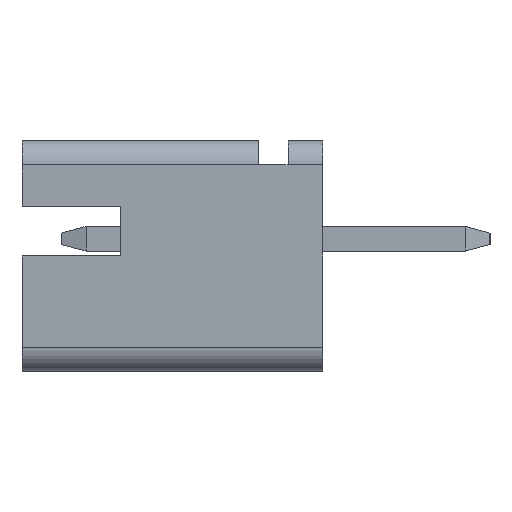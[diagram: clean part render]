
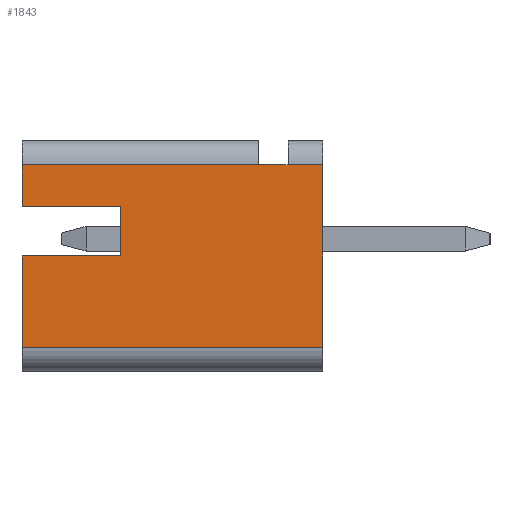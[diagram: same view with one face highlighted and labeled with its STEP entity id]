
A CAD part, left-side view. The second image highlights one B-rep face of the part: STEP entity #1843.
In plain terms, the highlighted planar face has unit normal (-1, 0, 0).
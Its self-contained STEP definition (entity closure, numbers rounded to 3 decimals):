
#8 = CARTESIAN_POINT ( 'NONE',  ( -2., 6.1, -0.35 ) ) ;
#12 = ORIENTED_EDGE ( 'NONE', *, *, #127, .F. ) ;
#119 = LINE ( 'NONE', #939, #4665 ) ;
#122 = VERTEX_POINT ( 'NONE', #4682 ) ;
#126 = CARTESIAN_POINT ( 'NONE',  ( -2., 0., 1.5 ) ) ;
#127 = EDGE_CURVE ( 'NONE', #3735, #2755, #2180, .T. ) ;
#175 = CARTESIAN_POINT ( 'NONE',  ( -2., 4.1, 0.65 ) ) ;
#351 = EDGE_CURVE ( 'NONE', #1900, #122, #1799, .T. ) ;
#388 = DIRECTION ( 'NONE',  ( 1., 0., 0. ) ) ;
#533 = VECTOR ( 'NONE', #1325, 1000. ) ;
#587 = DIRECTION ( 'NONE',  ( 0., -1., 0. ) ) ;
#600 = LINE ( 'NONE', #126, #533 ) ;
#610 = EDGE_CURVE ( 'NONE', #3731, #122, #5192, .T. ) ;
#653 = EDGE_CURVE ( 'NONE', #1260, #2563, #3970, .T. ) ;
#745 = CARTESIAN_POINT ( 'NONE',  ( -2., 1.3, 1.5 ) ) ;
#859 = CARTESIAN_POINT ( 'NONE',  ( -2., 6.1, -0.35 ) ) ;
#866 = VECTOR ( 'NONE', #4966, 1000. ) ;
#873 = CARTESIAN_POINT ( 'NONE',  ( -2., 6.1, -0.35 ) ) ;
#939 = CARTESIAN_POINT ( 'NONE',  ( -2., 6.1, 0.65 ) ) ;
#971 = DIRECTION ( 'NONE',  ( 0., 0., 1. ) ) ;
#1126 = FACE_OUTER_BOUND ( 'NONE', #1247, .T. ) ;
#1182 = DIRECTION ( 'NONE',  ( 0., 0., -1. ) ) ;
#1239 = LINE ( 'NONE', #1610, #4953 ) ;
#1240 = ORIENTED_EDGE ( 'NONE', *, *, #3850, .F. ) ;
#1247 = EDGE_LOOP ( 'NONE', ( #4267, #1818, #4338, #2055, #1240, #2957, #4111, #1693, #12, #4968 ) ) ;
#1260 = VERTEX_POINT ( 'NONE', #3298 ) ;
#1325 = DIRECTION ( 'NONE',  ( 0., 1., 0. ) ) ;
#1337 = CARTESIAN_POINT ( 'NONE',  ( -2., 0., 1.5 ) ) ;
#1405 = VECTOR ( 'NONE', #2483, 1000. ) ;
#1610 = CARTESIAN_POINT ( 'NONE',  ( -2., 0., 1.5 ) ) ;
#1614 = CARTESIAN_POINT ( 'NONE',  ( -2., 0., 2. ) ) ;
#1666 = LINE ( 'NONE', #873, #1405 ) ;
#1693 = ORIENTED_EDGE ( 'NONE', *, *, #3448, .F. ) ;
#1753 = LINE ( 'NONE', #859, #866 ) ;
#1758 = DIRECTION ( 'NONE',  ( 0., 1., 0. ) ) ;
#1799 = LINE ( 'NONE', #4664, #3803 ) ;
#1818 = ORIENTED_EDGE ( 'NONE', *, *, #351, .T. ) ;
#1843 = ADVANCED_FACE ( 'NONE', ( #1126 ), #2819, .F. ) ;
#1850 = LINE ( 'NONE', #4279, #2650 ) ;
#1900 = VERTEX_POINT ( 'NONE', #2023 ) ;
#2023 = CARTESIAN_POINT ( 'NONE',  ( -2., 6.1, -2.2 ) ) ;
#2055 = ORIENTED_EDGE ( 'NONE', *, *, #4324, .T. ) ;
#2180 = LINE ( 'NONE', #175, #3264 ) ;
#2277 = VECTOR ( 'NONE', #3176, 1000. ) ;
#2364 = VERTEX_POINT ( 'NONE', #2519 ) ;
#2483 = DIRECTION ( 'NONE',  ( 0., -1., 0. ) ) ;
#2519 = CARTESIAN_POINT ( 'NONE',  ( -2., 0.7, 1.5 ) ) ;
#2540 = VECTOR ( 'NONE', #3229, 1000. ) ;
#2563 = VERTEX_POINT ( 'NONE', #2581 ) ;
#2564 = EDGE_CURVE ( 'NONE', #4037, #2563, #600, .T. ) ;
#2581 = CARTESIAN_POINT ( 'NONE',  ( -2., 6.1, 1.5 ) ) ;
#2595 = DIRECTION ( 'NONE',  ( 0., -1., 0. ) ) ;
#2650 = VECTOR ( 'NONE', #2595, 1000. ) ;
#2660 = CARTESIAN_POINT ( 'NONE',  ( -2., 4.1, 0.65 ) ) ;
#2755 = VERTEX_POINT ( 'NONE', #2660 ) ;
#2819 = PLANE ( 'NONE',  #4036 ) ;
#2957 = ORIENTED_EDGE ( 'NONE', *, *, #2564, .T. ) ;
#3033 = EDGE_CURVE ( 'NONE', #4856, #3735, #1666, .T. ) ;
#3176 = DIRECTION ( 'NONE',  ( 0., 0., 1. ) ) ;
#3229 = DIRECTION ( 'NONE',  ( 0., 0., -1. ) ) ;
#3264 = VECTOR ( 'NONE', #971, 1000. ) ;
#3298 = CARTESIAN_POINT ( 'NONE',  ( -2., 6.1, 0.65 ) ) ;
#3448 = EDGE_CURVE ( 'NONE', #2755, #1260, #119, .T. ) ;
#3630 = EDGE_CURVE ( 'NONE', #1900, #4856, #1753, .T. ) ;
#3731 = VERTEX_POINT ( 'NONE', #1337 ) ;
#3735 = VERTEX_POINT ( 'NONE', #4095 ) ;
#3803 = VECTOR ( 'NONE', #587, 1000. ) ;
#3850 = EDGE_CURVE ( 'NONE', #4037, #2364, #1850, .T. ) ;
#3970 = LINE ( 'NONE', #4030, #2277 ) ;
#4030 = CARTESIAN_POINT ( 'NONE',  ( -2., 6.1, 2. ) ) ;
#4036 = AXIS2_PLACEMENT_3D ( 'NONE', #4431, #388, #1182 ) ;
#4037 = VERTEX_POINT ( 'NONE', #745 ) ;
#4095 = CARTESIAN_POINT ( 'NONE',  ( -2., 4.1, -0.35 ) ) ;
#4111 = ORIENTED_EDGE ( 'NONE', *, *, #653, .F. ) ;
#4267 = ORIENTED_EDGE ( 'NONE', *, *, #3630, .F. ) ;
#4279 = CARTESIAN_POINT ( 'NONE',  ( -2., 1.3, 1.5 ) ) ;
#4324 = EDGE_CURVE ( 'NONE', #3731, #2364, #1239, .T. ) ;
#4338 = ORIENTED_EDGE ( 'NONE', *, *, #610, .F. ) ;
#4431 = CARTESIAN_POINT ( 'NONE',  ( -2., 0., 0. ) ) ;
#4501 = DIRECTION ( 'NONE',  ( 0., 1., 0. ) ) ;
#4664 = CARTESIAN_POINT ( 'NONE',  ( -2., 0., -2.2 ) ) ;
#4665 = VECTOR ( 'NONE', #1758, 1000. ) ;
#4682 = CARTESIAN_POINT ( 'NONE',  ( -2., 0., -2.2 ) ) ;
#4856 = VERTEX_POINT ( 'NONE', #8 ) ;
#4953 = VECTOR ( 'NONE', #4501, 1000. ) ;
#4966 = DIRECTION ( 'NONE',  ( 0., 0., 1. ) ) ;
#4968 = ORIENTED_EDGE ( 'NONE', *, *, #3033, .F. ) ;
#5192 = LINE ( 'NONE', #1614, #2540 ) ;
